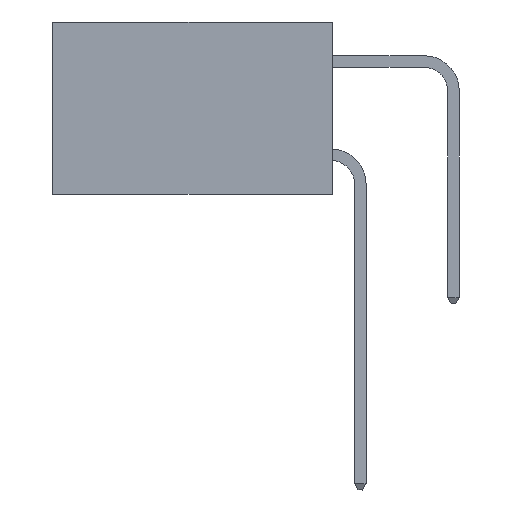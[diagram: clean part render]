
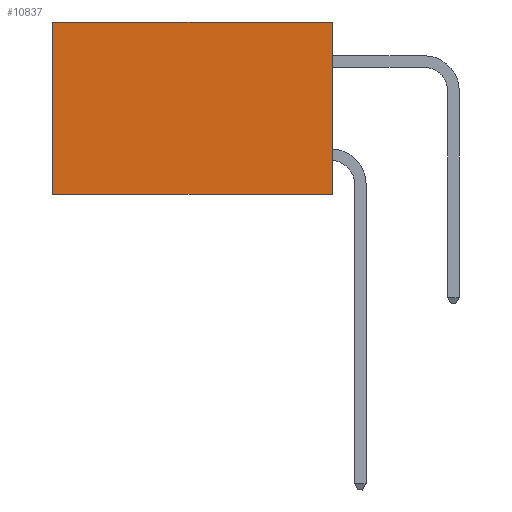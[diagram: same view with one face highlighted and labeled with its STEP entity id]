
A CAD part, left-side view. The second image highlights one B-rep face of the part: STEP entity #10837.
In plain terms, the highlighted planar face has unit normal (-1, 0, 0).
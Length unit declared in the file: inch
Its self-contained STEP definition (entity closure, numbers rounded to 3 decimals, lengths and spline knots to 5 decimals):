
#152 = LINE ( 'NONE', #16158, #4539 ) ;
#534 = DIRECTION ( 'NONE',  ( 0., 0., -1. ) ) ;
#717 = CARTESIAN_POINT ( 'NONE',  ( 0.2615, 0., -0.37 ) ) ;
#1536 = AXIS2_PLACEMENT_3D ( 'NONE', #1548, #12979, #9817 ) ;
#1548 = CARTESIAN_POINT ( 'NONE',  ( 0.2615, 0., -0.37 ) ) ;
#1814 = LINE ( 'NONE', #12364, #14942 ) ;
#2380 = CARTESIAN_POINT ( 'NONE',  ( 0.2615, 0., 0. ) ) ;
#2913 = DIRECTION ( 'NONE',  ( 0., 1., 0. ) ) ;
#3624 = VECTOR ( 'NONE', #534, 39.37008 ) ;
#3788 = LINE ( 'NONE', #2380, #14741 ) ;
#4539 = VECTOR ( 'NONE', #2913, 39.37008 ) ;
#4618 = CARTESIAN_POINT ( 'NONE',  ( 0.2615, 0.6, 0. ) ) ;
#5720 = ORIENTED_EDGE ( 'NONE', *, *, #6970, .F. ) ;
#5797 = ORIENTED_EDGE ( 'NONE', *, *, #9743, .T. ) ;
#6440 = VERTEX_POINT ( 'NONE', #7987 ) ;
#6798 = EDGE_LOOP ( 'NONE', ( #5797, #5720, #18318, #11673 ) ) ;
#6956 = VERTEX_POINT ( 'NONE', #13102 ) ;
#6970 = EDGE_CURVE ( 'NONE', #6956, #11723, #152, .T. ) ;
#7071 = VERTEX_POINT ( 'NONE', #4618 ) ;
#7987 = CARTESIAN_POINT ( 'NONE',  ( 0.2615, 0., 0. ) ) ;
#8528 = EDGE_CURVE ( 'NONE', #6440, #6956, #15191, .T. ) ;
#9743 = EDGE_CURVE ( 'NONE', #7071, #11723, #1814, .T. ) ;
#9817 = DIRECTION ( 'NONE',  ( 0., 0., -1. ) ) ;
#10837 = ADVANCED_FACE ( 'NONE', ( #14603 ), #16030, .F. ) ;
#11123 = DIRECTION ( 'NONE',  ( 0., 1., 0. ) ) ;
#11673 = ORIENTED_EDGE ( 'NONE', *, *, #17293, .T. ) ;
#11723 = VERTEX_POINT ( 'NONE', #14532 ) ;
#12272 = DIRECTION ( 'NONE',  ( 0., 0., -1. ) ) ;
#12364 = CARTESIAN_POINT ( 'NONE',  ( 0.2615, 0.6, -0.37 ) ) ;
#12979 = DIRECTION ( 'NONE',  ( 1., 0., 0. ) ) ;
#13102 = CARTESIAN_POINT ( 'NONE',  ( 0.2615, 0., -0.37 ) ) ;
#14532 = CARTESIAN_POINT ( 'NONE',  ( 0.2615, 0.6, -0.37 ) ) ;
#14603 = FACE_OUTER_BOUND ( 'NONE', #6798, .T. ) ;
#14741 = VECTOR ( 'NONE', #11123, 39.37008 ) ;
#14942 = VECTOR ( 'NONE', #12272, 39.37008 ) ;
#15191 = LINE ( 'NONE', #717, #3624 ) ;
#16030 = PLANE ( 'NONE',  #1536 ) ;
#16158 = CARTESIAN_POINT ( 'NONE',  ( 0.2615, 0., -0.37 ) ) ;
#17293 = EDGE_CURVE ( 'NONE', #6440, #7071, #3788, .T. ) ;
#18318 = ORIENTED_EDGE ( 'NONE', *, *, #8528, .F. ) ;
